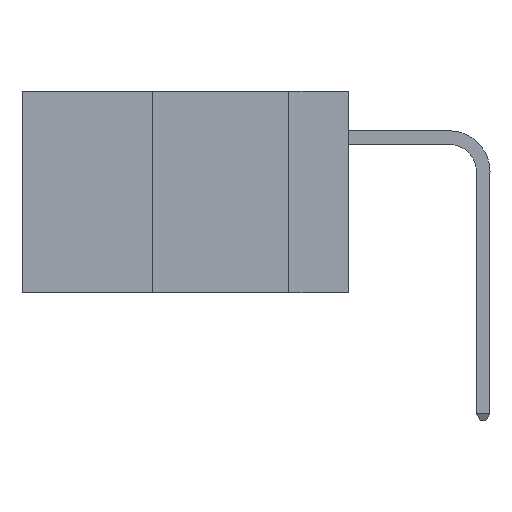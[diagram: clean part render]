
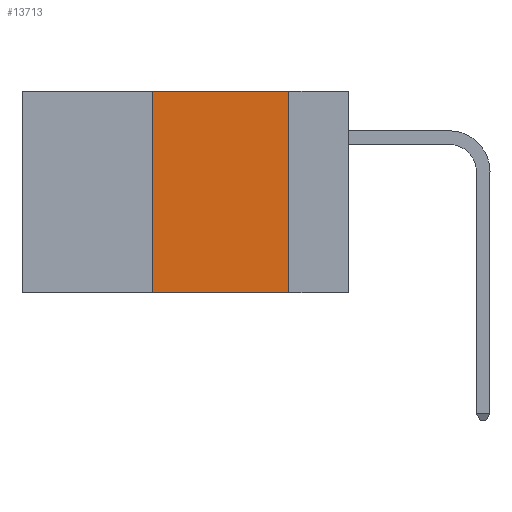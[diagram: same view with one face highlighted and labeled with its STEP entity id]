
A CAD part, left-side view. The second image highlights one B-rep face of the part: STEP entity #13713.
In plain terms, the highlighted planar face has unit normal (-1, 0, 0).
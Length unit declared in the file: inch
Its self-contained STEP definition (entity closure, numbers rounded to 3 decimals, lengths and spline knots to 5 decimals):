
#33 = LINE ( 'NONE', #1525, #10099 ) ;
#84 = EDGE_CURVE ( 'NONE', #3714, #6559, #33, .T. ) ;
#85 = EDGE_CURVE ( 'NONE', #2206, #386, #12470, .T. ) ;
#166 = DIRECTION ( 'NONE',  ( 0., -1., 0. ) ) ;
#386 = VERTEX_POINT ( 'NONE', #918 ) ;
#577 = CARTESIAN_POINT ( 'NONE',  ( 0., 0.11, 0. ) ) ;
#918 = CARTESIAN_POINT ( 'NONE',  ( 0., 0.11, -0.37 ) ) ;
#1525 = CARTESIAN_POINT ( 'NONE',  ( 0., 0.6, 0. ) ) ;
#1637 = EDGE_CURVE ( 'NONE', #6559, #386, #6429, .T. ) ;
#2206 = VERTEX_POINT ( 'NONE', #3878 ) ;
#2837 = PLANE ( 'NONE',  #18748 ) ;
#2909 = DIRECTION ( 'NONE',  ( 1., 0., 0. ) ) ;
#3338 = CARTESIAN_POINT ( 'NONE',  ( 0., 0.6, -0.37 ) ) ;
#3714 = VERTEX_POINT ( 'NONE', #13413 ) ;
#3878 = CARTESIAN_POINT ( 'NONE',  ( 0., 0.36, -0.37 ) ) ;
#4054 = VECTOR ( 'NONE', #15260, 39.37008 ) ;
#4358 = CARTESIAN_POINT ( 'NONE',  ( 0., 0.6, 0. ) ) ;
#5508 = FACE_OUTER_BOUND ( 'NONE', #18087, .T. ) ;
#5751 = ORIENTED_EDGE ( 'NONE', *, *, #1637, .F. ) ;
#5934 = DIRECTION ( 'NONE',  ( 0., 0., -1. ) ) ;
#6389 = CARTESIAN_POINT ( 'NONE',  ( 0., 0.36, 0. ) ) ;
#6429 = LINE ( 'NONE', #577, #12461 ) ;
#6518 = ORIENTED_EDGE ( 'NONE', *, *, #13095, .F. ) ;
#6559 = VERTEX_POINT ( 'NONE', #10555 ) ;
#7628 = DIRECTION ( 'NONE',  ( 0., 0., -1. ) ) ;
#9627 = ORIENTED_EDGE ( 'NONE', *, *, #85, .T. ) ;
#10099 = VECTOR ( 'NONE', #166, 39.37008 ) ;
#10555 = CARTESIAN_POINT ( 'NONE',  ( 0., 0.11, 0. ) ) ;
#12431 = LINE ( 'NONE', #6389, #15494 ) ;
#12461 = VECTOR ( 'NONE', #7628, 39.37008 ) ;
#12470 = LINE ( 'NONE', #3338, #4054 ) ;
#13095 = EDGE_CURVE ( 'NONE', #2206, #3714, #12431, .T. ) ;
#13413 = CARTESIAN_POINT ( 'NONE',  ( 0., 0.36, 0. ) ) ;
#13713 = ADVANCED_FACE ( 'NONE', ( #5508 ), #2837, .F. ) ;
#15260 = DIRECTION ( 'NONE',  ( 0., -1., 0. ) ) ;
#15494 = VECTOR ( 'NONE', #16810, 39.37008 ) ;
#16810 = DIRECTION ( 'NONE',  ( 0., 0., 1. ) ) ;
#17438 = ORIENTED_EDGE ( 'NONE', *, *, #84, .F. ) ;
#18087 = EDGE_LOOP ( 'NONE', ( #5751, #17438, #6518, #9627 ) ) ;
#18748 = AXIS2_PLACEMENT_3D ( 'NONE', #4358, #2909, #5934 ) ;
